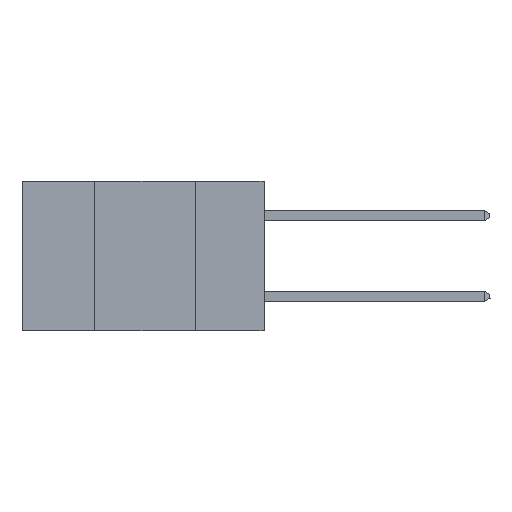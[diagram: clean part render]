
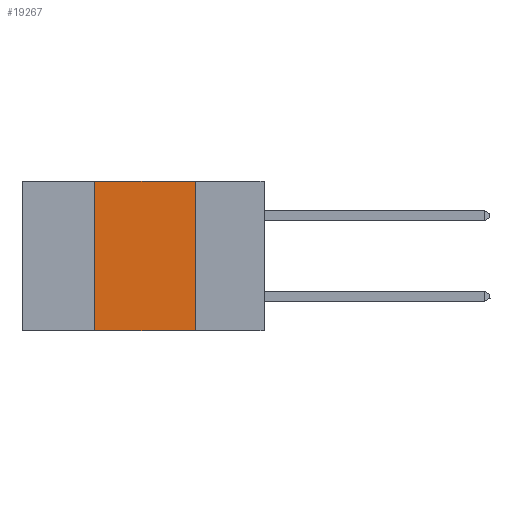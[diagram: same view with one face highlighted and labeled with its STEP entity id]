
A CAD part, left-side view. The second image highlights one B-rep face of the part: STEP entity #19267.
In plain terms, the highlighted planar face has unit normal (-1, 0, 0).
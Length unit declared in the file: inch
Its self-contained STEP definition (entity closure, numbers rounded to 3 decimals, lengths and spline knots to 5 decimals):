
#553 = VECTOR ( 'NONE', #25810, 39.37008 ) ;
#1020 = AXIS2_PLACEMENT_3D ( 'NONE', #16525, #7853, #23016 ) ;
#1541 = CARTESIAN_POINT ( 'NONE',  ( 0., 0.17, 0. ) ) ;
#1734 = DIRECTION ( 'NONE',  ( 0., -1., 0. ) ) ;
#2641 = EDGE_CURVE ( 'NONE', #16993, #4158, #15671, .T. ) ;
#3984 = EDGE_CURVE ( 'NONE', #8251, #4158, #9095, .T. ) ;
#3995 = CARTESIAN_POINT ( 'NONE',  ( 0., 0.17, 0. ) ) ;
#4158 = VERTEX_POINT ( 'NONE', #5568 ) ;
#4251 = EDGE_CURVE ( 'NONE', #21619, #16993, #26634, .T. ) ;
#4326 = ORIENTED_EDGE ( 'NONE', *, *, #4251, .F. ) ;
#5568 = CARTESIAN_POINT ( 'NONE',  ( 0., 0.17, -0.37 ) ) ;
#5811 = LINE ( 'NONE', #10710, #553 ) ;
#6170 = FACE_OUTER_BOUND ( 'NONE', #25491, .T. ) ;
#7853 = DIRECTION ( 'NONE',  ( 1., 0., 0. ) ) ;
#8251 = VERTEX_POINT ( 'NONE', #11730 ) ;
#9095 = LINE ( 'NONE', #23193, #14908 ) ;
#10710 = CARTESIAN_POINT ( 'NONE',  ( 0., 0.42, 0. ) ) ;
#11730 = CARTESIAN_POINT ( 'NONE',  ( 0., 0.42, -0.37 ) ) ;
#13890 = ORIENTED_EDGE ( 'NONE', *, *, #3984, .T. ) ;
#14908 = VECTOR ( 'NONE', #1734, 39.37008 ) ;
#14988 = VECTOR ( 'NONE', #21823, 39.37008 ) ;
#15480 = CARTESIAN_POINT ( 'NONE',  ( 0., 0.6, 0. ) ) ;
#15671 = LINE ( 'NONE', #1541, #14988 ) ;
#16104 = ORIENTED_EDGE ( 'NONE', *, *, #2641, .F. ) ;
#16417 = CARTESIAN_POINT ( 'NONE',  ( 0., 0.42, 0. ) ) ;
#16525 = CARTESIAN_POINT ( 'NONE',  ( 0., 0.6, 0. ) ) ;
#16993 = VERTEX_POINT ( 'NONE', #3995 ) ;
#19267 = ADVANCED_FACE ( 'NONE', ( #6170 ), #20868, .F. ) ;
#20868 = PLANE ( 'NONE',  #1020 ) ;
#21619 = VERTEX_POINT ( 'NONE', #16417 ) ;
#21823 = DIRECTION ( 'NONE',  ( 0., 0., -1. ) ) ;
#22678 = ORIENTED_EDGE ( 'NONE', *, *, #26182, .F. ) ;
#23016 = DIRECTION ( 'NONE',  ( 0., 0., -1. ) ) ;
#23193 = CARTESIAN_POINT ( 'NONE',  ( 0., 0.6, -0.37 ) ) ;
#25316 = VECTOR ( 'NONE', #26216, 39.37008 ) ;
#25491 = EDGE_LOOP ( 'NONE', ( #16104, #4326, #22678, #13890 ) ) ;
#25810 = DIRECTION ( 'NONE',  ( 0., 0., 1. ) ) ;
#26182 = EDGE_CURVE ( 'NONE', #8251, #21619, #5811, .T. ) ;
#26216 = DIRECTION ( 'NONE',  ( 0., -1., 0. ) ) ;
#26634 = LINE ( 'NONE', #15480, #25316 ) ;
